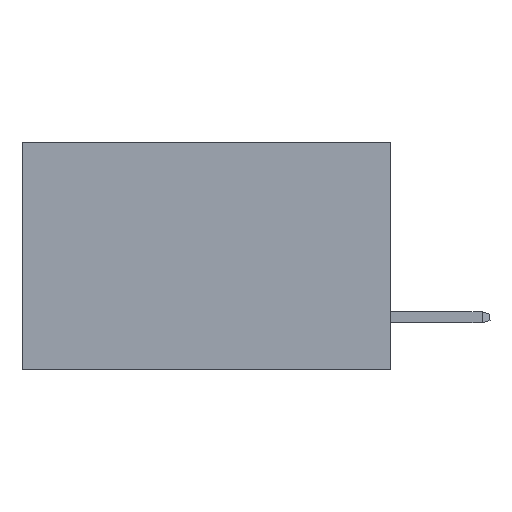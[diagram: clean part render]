
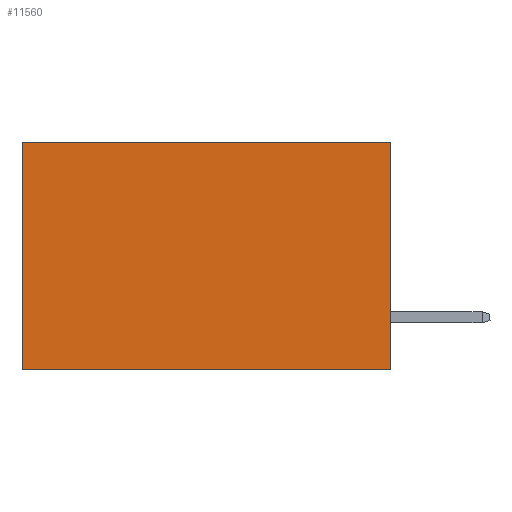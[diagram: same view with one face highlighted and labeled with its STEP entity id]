
A CAD part, left-side view. The second image highlights one B-rep face of the part: STEP entity #11560.
In plain terms, the highlighted planar face has unit normal (-1, 0, 0).
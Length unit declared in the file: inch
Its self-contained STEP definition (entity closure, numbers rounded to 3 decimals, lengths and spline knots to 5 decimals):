
#39 = EDGE_CURVE ( 'NONE', #4617, #12936, #10151, .T. ) ;
#361 = LINE ( 'NONE', #11429, #4181 ) ;
#1207 = ORIENTED_EDGE ( 'NONE', *, *, #2674, .T. ) ;
#1286 = CARTESIAN_POINT ( 'NONE',  ( 0.2875, 0., -0.37 ) ) ;
#2674 = EDGE_CURVE ( 'NONE', #12851, #5613, #11983, .T. ) ;
#3029 = DIRECTION ( 'NONE',  ( 0., 0., -1. ) ) ;
#3371 = CARTESIAN_POINT ( 'NONE',  ( 0.2875, 0.6, 0. ) ) ;
#3456 = DIRECTION ( 'NONE',  ( 0., 1., 0. ) ) ;
#4159 = PLANE ( 'NONE',  #12712 ) ;
#4181 = VECTOR ( 'NONE', #3456, 39.37008 ) ;
#4268 = FACE_OUTER_BOUND ( 'NONE', #8228, .T. ) ;
#4617 = VERTEX_POINT ( 'NONE', #11861 ) ;
#4674 = VECTOR ( 'NONE', #12301, 39.37008 ) ;
#5310 = DIRECTION ( 'NONE',  ( 0., 0., -1. ) ) ;
#5448 = CARTESIAN_POINT ( 'NONE',  ( 0.2875, 0., -0.37 ) ) ;
#5613 = VERTEX_POINT ( 'NONE', #11030 ) ;
#6000 = ORIENTED_EDGE ( 'NONE', *, *, #9923, .F. ) ;
#6772 = ORIENTED_EDGE ( 'NONE', *, *, #39, .F. ) ;
#7055 = VECTOR ( 'NONE', #14401, 39.37008 ) ;
#8228 = EDGE_LOOP ( 'NONE', ( #1207, #6000, #6772, #12545 ) ) ;
#8802 = CARTESIAN_POINT ( 'NONE',  ( 0.2875, 0., 0. ) ) ;
#9377 = VECTOR ( 'NONE', #3029, 39.37008 ) ;
#9404 = EDGE_CURVE ( 'NONE', #4617, #12851, #361, .T. ) ;
#9923 = EDGE_CURVE ( 'NONE', #12936, #5613, #10824, .T. ) ;
#10151 = LINE ( 'NONE', #14303, #7055 ) ;
#10824 = LINE ( 'NONE', #5448, #4674 ) ;
#11030 = CARTESIAN_POINT ( 'NONE',  ( 0.2875, 0.6, -0.37 ) ) ;
#11429 = CARTESIAN_POINT ( 'NONE',  ( 0.2875, 0., 0. ) ) ;
#11560 = ADVANCED_FACE ( 'NONE', ( #4268 ), #4159, .F. ) ;
#11861 = CARTESIAN_POINT ( 'NONE',  ( 0.2875, 0., 0. ) ) ;
#11983 = LINE ( 'NONE', #3371, #9377 ) ;
#12164 = DIRECTION ( 'NONE',  ( 1., 0., 0. ) ) ;
#12301 = DIRECTION ( 'NONE',  ( 0., 1., 0. ) ) ;
#12545 = ORIENTED_EDGE ( 'NONE', *, *, #9404, .T. ) ;
#12574 = CARTESIAN_POINT ( 'NONE',  ( 0.2875, 0.6, 0. ) ) ;
#12712 = AXIS2_PLACEMENT_3D ( 'NONE', #8802, #12164, #5310 ) ;
#12851 = VERTEX_POINT ( 'NONE', #12574 ) ;
#12936 = VERTEX_POINT ( 'NONE', #1286 ) ;
#14303 = CARTESIAN_POINT ( 'NONE',  ( 0.2875, 0., 0. ) ) ;
#14401 = DIRECTION ( 'NONE',  ( 0., 0., -1. ) ) ;
